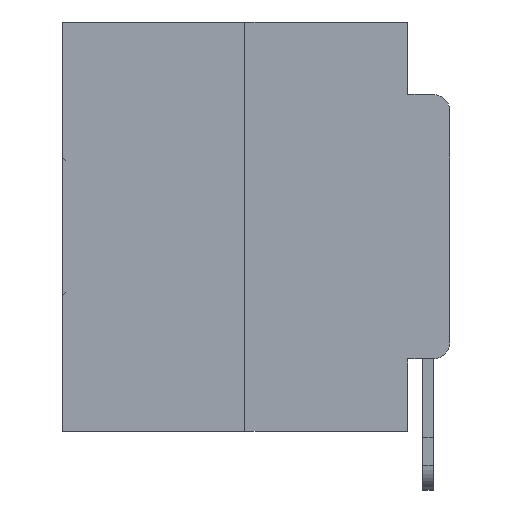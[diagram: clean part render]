
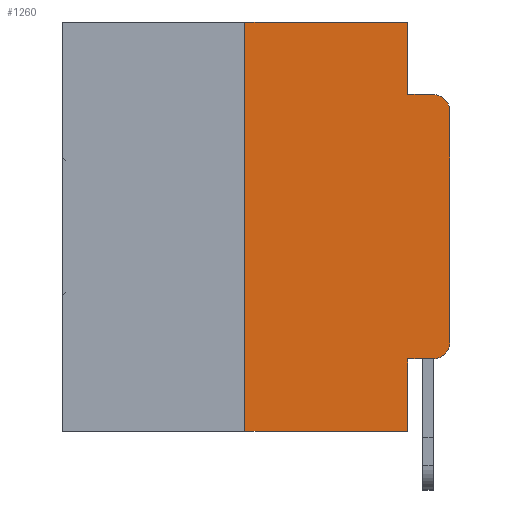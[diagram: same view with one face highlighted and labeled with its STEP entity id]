
A CAD part, left-side view. The second image highlights one B-rep face of the part: STEP entity #1260.
In plain terms, the highlighted planar face has unit normal (-1, 0, 0).
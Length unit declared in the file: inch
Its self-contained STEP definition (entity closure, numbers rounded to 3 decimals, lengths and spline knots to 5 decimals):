
#80 = LINE ( 'NONE', #9434, #12937 ) ;
#659 = CARTESIAN_POINT ( 'NONE',  ( 0., 0.02, -0.1085 ) ) ;
#795 = LINE ( 'NONE', #22056, #25654 ) ;
#1260 = ADVANCED_FACE ( 'NONE', ( #29094 ), #14503, .F. ) ;
#1719 = CARTESIAN_POINT ( 'NONE',  ( 0., 0.25, 0. ) ) ;
#1967 = DIRECTION ( 'NONE',  ( 1., 0., 0. ) ) ;
#2046 = EDGE_CURVE ( 'NONE', #13616, #3334, #26209, .T. ) ;
#2315 = VERTEX_POINT ( 'NONE', #25468 ) ;
#2554 = DIRECTION ( 'NONE',  ( 0., -1., 0. ) ) ;
#2915 = VERTEX_POINT ( 'NONE', #1719 ) ;
#2996 = CARTESIAN_POINT ( 'NONE',  ( 0., 0.02, -0.4115 ) ) ;
#3334 = VERTEX_POINT ( 'NONE', #2996 ) ;
#3355 = DIRECTION ( 'NONE',  ( 0., 0., -1. ) ) ;
#4684 = VECTOR ( 'NONE', #2554, 39.37008 ) ;
#5029 = CARTESIAN_POINT ( 'NONE',  ( 0., 0.25, 0. ) ) ;
#5141 = CARTESIAN_POINT ( 'NONE',  ( 0., 0., 0. ) ) ;
#5251 = DIRECTION ( 'NONE',  ( 0., 0., 1. ) ) ;
#5280 = DIRECTION ( 'NONE',  ( -1., 0., 0. ) ) ;
#6792 = VECTOR ( 'NONE', #22225, 39.37008 ) ;
#6804 = AXIS2_PLACEMENT_3D ( 'NONE', #28009, #1967, #19096 ) ;
#6970 = AXIS2_PLACEMENT_3D ( 'NONE', #19680, #5280, #21972 ) ;
#7653 = DIRECTION ( 'NONE',  ( 0., 0., 1. ) ) ;
#8199 = EDGE_CURVE ( 'NONE', #2915, #30579, #28694, .T. ) ;
#9434 = CARTESIAN_POINT ( 'NONE',  ( 0., 0.051, 0. ) ) ;
#9564 = ORIENTED_EDGE ( 'NONE', *, *, #25911, .T. ) ;
#10550 = DIRECTION ( 'NONE',  ( 0., 0., -1. ) ) ;
#10634 = VECTOR ( 'NONE', #29075, 39.37008 ) ;
#11058 = VECTOR ( 'NONE', #7653, 39.37008 ) ;
#12937 = VECTOR ( 'NONE', #27888, 39.37008 ) ;
#13328 = CIRCLE ( 'NONE', #16342, 0.02 ) ;
#13616 = VERTEX_POINT ( 'NONE', #20352 ) ;
#14169 = CIRCLE ( 'NONE', #6970, 0.02 ) ;
#14214 = ORIENTED_EDGE ( 'NONE', *, *, #25352, .T. ) ;
#14503 = PLANE ( 'NONE',  #6804 ) ;
#14593 = ORIENTED_EDGE ( 'NONE', *, *, #25146, .F. ) ;
#14728 = VERTEX_POINT ( 'NONE', #19211 ) ;
#14833 = CARTESIAN_POINT ( 'NONE',  ( 0., 0.473, 0. ) ) ;
#15004 = EDGE_CURVE ( 'NONE', #2315, #14728, #16874, .T. ) ;
#15016 = CARTESIAN_POINT ( 'NONE',  ( 0., 0.051, -0.0885 ) ) ;
#15510 = CARTESIAN_POINT ( 'NONE',  ( 0., 0.473, -0.5 ) ) ;
#15572 = EDGE_CURVE ( 'NONE', #2315, #2915, #23290, .T. ) ;
#15926 = VECTOR ( 'NONE', #26230, 39.37008 ) ;
#16342 = AXIS2_PLACEMENT_3D ( 'NONE', #659, #18025, #3355 ) ;
#16799 = ORIENTED_EDGE ( 'NONE', *, *, #27735, .F. ) ;
#16874 = LINE ( 'NONE', #15510, #10634 ) ;
#17586 = CARTESIAN_POINT ( 'NONE',  ( 0., 0.051, -0.4115 ) ) ;
#18025 = DIRECTION ( 'NONE',  ( -1., 0., 0. ) ) ;
#18845 = VERTEX_POINT ( 'NONE', #27215 ) ;
#19096 = DIRECTION ( 'NONE',  ( 0., 0., -1. ) ) ;
#19211 = CARTESIAN_POINT ( 'NONE',  ( 0., 0.051, -0.5 ) ) ;
#19325 = ORIENTED_EDGE ( 'NONE', *, *, #15004, .T. ) ;
#19680 = CARTESIAN_POINT ( 'NONE',  ( 0., 0.02, -0.3915 ) ) ;
#20352 = CARTESIAN_POINT ( 'NONE',  ( 0., 0.051, -0.4115 ) ) ;
#20600 = ORIENTED_EDGE ( 'NONE', *, *, #23420, .T. ) ;
#20954 = ORIENTED_EDGE ( 'NONE', *, *, #2046, .T. ) ;
#21972 = DIRECTION ( 'NONE',  ( 0., 0., -1. ) ) ;
#22056 = CARTESIAN_POINT ( 'NONE',  ( 0., 0.051, 0. ) ) ;
#22225 = DIRECTION ( 'NONE',  ( 0., -1., 0. ) ) ;
#22327 = CARTESIAN_POINT ( 'NONE',  ( 0., 0.02, -0.0885 ) ) ;
#22682 = EDGE_LOOP ( 'NONE', ( #9564, #14214, #14593, #16799, #24969, #23690, #19325, #27676, #20954, #20600 ) ) ;
#23113 = CARTESIAN_POINT ( 'NONE',  ( 0., 0.051, -0.0885 ) ) ;
#23290 = LINE ( 'NONE', #5029, #11058 ) ;
#23420 = EDGE_CURVE ( 'NONE', #3334, #26263, #14169, .T. ) ;
#23690 = ORIENTED_EDGE ( 'NONE', *, *, #15572, .F. ) ;
#24633 = CARTESIAN_POINT ( 'NONE',  ( 0., 0.051, 0. ) ) ;
#24714 = LINE ( 'NONE', #5141, #29976 ) ;
#24969 = ORIENTED_EDGE ( 'NONE', *, *, #8199, .F. ) ;
#25146 = EDGE_CURVE ( 'NONE', #26638, #26345, #29651, .T. ) ;
#25352 = EDGE_CURVE ( 'NONE', #18845, #26345, #13328, .T. ) ;
#25468 = CARTESIAN_POINT ( 'NONE',  ( 0., 0.25, -0.5 ) ) ;
#25647 = EDGE_CURVE ( 'NONE', #13616, #14728, #80, .T. ) ;
#25654 = VECTOR ( 'NONE', #10550, 39.37008 ) ;
#25911 = EDGE_CURVE ( 'NONE', #26263, #18845, #24714, .T. ) ;
#26209 = LINE ( 'NONE', #17586, #6792 ) ;
#26230 = DIRECTION ( 'NONE',  ( 0., -1., 0. ) ) ;
#26263 = VERTEX_POINT ( 'NONE', #26574 ) ;
#26345 = VERTEX_POINT ( 'NONE', #22327 ) ;
#26574 = CARTESIAN_POINT ( 'NONE',  ( 0., 0., -0.3915 ) ) ;
#26638 = VERTEX_POINT ( 'NONE', #23113 ) ;
#27215 = CARTESIAN_POINT ( 'NONE',  ( 0., 0., -0.1085 ) ) ;
#27676 = ORIENTED_EDGE ( 'NONE', *, *, #25647, .F. ) ;
#27735 = EDGE_CURVE ( 'NONE', #30579, #26638, #795, .T. ) ;
#27888 = DIRECTION ( 'NONE',  ( 0., 0., -1. ) ) ;
#28009 = CARTESIAN_POINT ( 'NONE',  ( 0., 0.473, 0. ) ) ;
#28694 = LINE ( 'NONE', #14833, #15926 ) ;
#29075 = DIRECTION ( 'NONE',  ( 0., -1., 0. ) ) ;
#29094 = FACE_OUTER_BOUND ( 'NONE', #22682, .T. ) ;
#29651 = LINE ( 'NONE', #15016, #4684 ) ;
#29976 = VECTOR ( 'NONE', #5251, 39.37008 ) ;
#30579 = VERTEX_POINT ( 'NONE', #24633 ) ;
